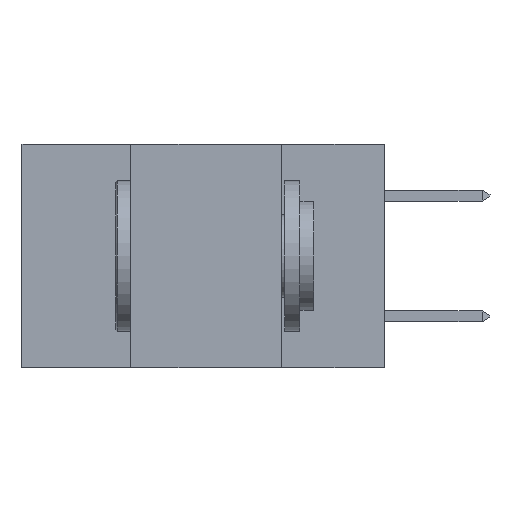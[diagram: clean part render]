
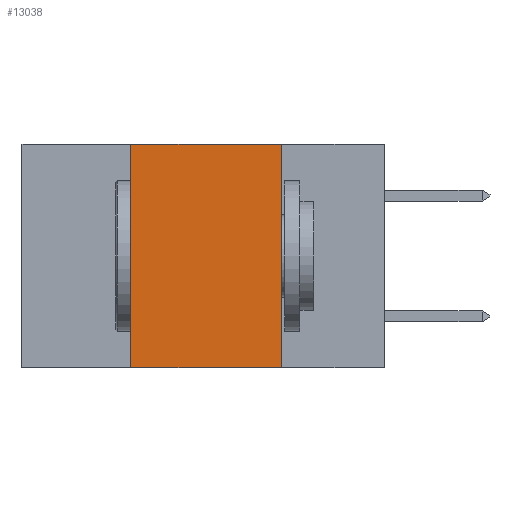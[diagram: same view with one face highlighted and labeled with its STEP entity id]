
A CAD part, left-side view. The second image highlights one B-rep face of the part: STEP entity #13038.
In plain terms, the highlighted planar face has unit normal (-1, 0, 0).
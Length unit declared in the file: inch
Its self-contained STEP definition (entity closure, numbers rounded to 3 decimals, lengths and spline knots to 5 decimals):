
#1146 = DIRECTION ( 'NONE',  ( 0., 0., 1. ) ) ;
#1246 = LINE ( 'NONE', #5025, #15374 ) ;
#1771 = LINE ( 'NONE', #11345, #9942 ) ;
#2256 = CARTESIAN_POINT ( 'NONE',  ( 0., 0.6, -0.37 ) ) ;
#2438 = CARTESIAN_POINT ( 'NONE',  ( 0., 0.42, -0.37 ) ) ;
#4121 = CARTESIAN_POINT ( 'NONE',  ( 0., 0.17, -0.37 ) ) ;
#4428 = CARTESIAN_POINT ( 'NONE',  ( 0., 0.42, 0. ) ) ;
#4535 = VERTEX_POINT ( 'NONE', #12022 ) ;
#5025 = CARTESIAN_POINT ( 'NONE',  ( 0., 0.6, 0. ) ) ;
#5240 = ORIENTED_EDGE ( 'NONE', *, *, #7192, .T. ) ;
#5461 = FACE_OUTER_BOUND ( 'NONE', #8432, .T. ) ;
#6901 = LINE ( 'NONE', #2256, #11011 ) ;
#7192 = EDGE_CURVE ( 'NONE', #13845, #21367, #6901, .T. ) ;
#7445 = EDGE_CURVE ( 'NONE', #9696, #4535, #1246, .T. ) ;
#8432 = EDGE_LOOP ( 'NONE', ( #20428, #22489, #14688, #5240 ) ) ;
#9040 = PLANE ( 'NONE',  #18786 ) ;
#9064 = DIRECTION ( 'NONE',  ( 0., -1., 0. ) ) ;
#9696 = VERTEX_POINT ( 'NONE', #4428 ) ;
#9942 = VECTOR ( 'NONE', #1146, 39.37008 ) ;
#10511 = EDGE_CURVE ( 'NONE', #4535, #21367, #22809, .T. ) ;
#11011 = VECTOR ( 'NONE', #12867, 39.37008 ) ;
#11345 = CARTESIAN_POINT ( 'NONE',  ( 0., 0.42, 0. ) ) ;
#12022 = CARTESIAN_POINT ( 'NONE',  ( 0., 0.17, 0. ) ) ;
#12867 = DIRECTION ( 'NONE',  ( 0., -1., 0. ) ) ;
#13038 = ADVANCED_FACE ( 'NONE', ( #5461 ), #9040, .F. ) ;
#13845 = VERTEX_POINT ( 'NONE', #2438 ) ;
#14260 = DIRECTION ( 'NONE',  ( 0., 0., -1. ) ) ;
#14688 = ORIENTED_EDGE ( 'NONE', *, *, #19827, .F. ) ;
#14766 = DIRECTION ( 'NONE',  ( 1., 0., 0. ) ) ;
#15031 = CARTESIAN_POINT ( 'NONE',  ( 0., 0.6, 0. ) ) ;
#15374 = VECTOR ( 'NONE', #9064, 39.37008 ) ;
#16887 = DIRECTION ( 'NONE',  ( 0., 0., -1. ) ) ;
#18786 = AXIS2_PLACEMENT_3D ( 'NONE', #15031, #14766, #16887 ) ;
#19827 = EDGE_CURVE ( 'NONE', #13845, #9696, #1771, .T. ) ;
#20428 = ORIENTED_EDGE ( 'NONE', *, *, #10511, .F. ) ;
#21367 = VERTEX_POINT ( 'NONE', #4121 ) ;
#22455 = CARTESIAN_POINT ( 'NONE',  ( 0., 0.17, 0. ) ) ;
#22489 = ORIENTED_EDGE ( 'NONE', *, *, #7445, .F. ) ;
#22809 = LINE ( 'NONE', #22455, #24698 ) ;
#24698 = VECTOR ( 'NONE', #14260, 39.37008 ) ;
